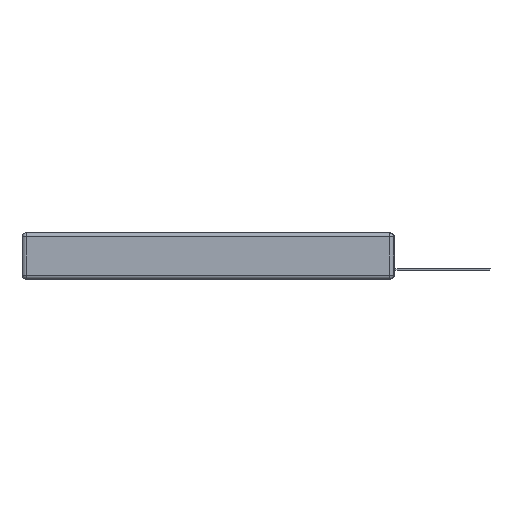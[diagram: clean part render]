
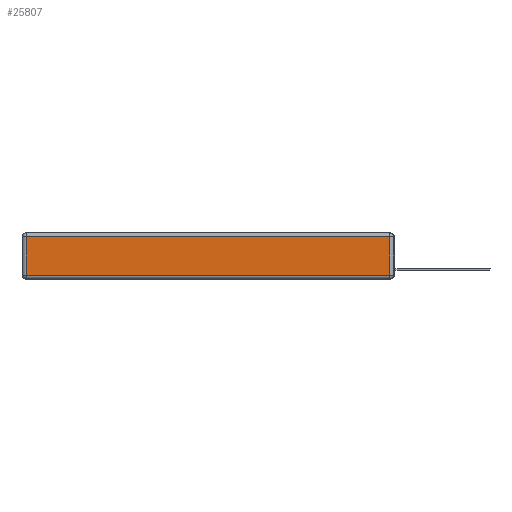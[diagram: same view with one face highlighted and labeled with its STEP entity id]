
A CAD part, left-side view. The second image highlights one B-rep face of the part: STEP entity #25807.
In plain terms, the highlighted planar face has unit normal (-1, 0, 0).
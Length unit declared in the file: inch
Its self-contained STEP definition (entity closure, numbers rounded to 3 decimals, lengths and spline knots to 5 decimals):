
#440 = DIRECTION ( 'NONE',  ( -1., 0., 0. ) ) ;
#2478 = PLANE ( 'NONE',  #12791 ) ;
#2831 = EDGE_CURVE ( 'NONE', #24040, #21944, #13257, .T. ) ;
#2901 = VERTEX_POINT ( 'NONE', #25821 ) ;
#3706 = VERTEX_POINT ( 'NONE', #24726 ) ;
#4555 = EDGE_CURVE ( 'NONE', #3706, #2901, #20381, .T. ) ;
#4625 = DIRECTION ( 'NONE',  ( 0., -1., 0. ) ) ;
#4902 = EDGE_CURVE ( 'NONE', #21944, #3706, #15594, .T. ) ;
#4913 = FACE_OUTER_BOUND ( 'NONE', #13018, .T. ) ;
#5460 = CARTESIAN_POINT ( 'NONE',  ( 0., 2.72, -0.343 ) ) ;
#5959 = VECTOR ( 'NONE', #4625, 39.37008 ) ;
#6176 = DIRECTION ( 'NONE',  ( 0., 1., 0. ) ) ;
#6598 = CARTESIAN_POINT ( 'NONE',  ( 0., 2.72, -0.313 ) ) ;
#7191 = ORIENTED_EDGE ( 'NONE', *, *, #4902, .T. ) ;
#12208 = VECTOR ( 'NONE', #6176, 39.37008 ) ;
#12253 = ORIENTED_EDGE ( 'NONE', *, *, #2831, .T. ) ;
#12481 = ORIENTED_EDGE ( 'NONE', *, *, #18104, .T. ) ;
#12791 = AXIS2_PLACEMENT_3D ( 'NONE', #19145, #440, #17092 ) ;
#12843 = CARTESIAN_POINT ( 'NONE',  ( 0., 0., -0.313 ) ) ;
#13018 = EDGE_LOOP ( 'NONE', ( #12253, #7191, #16410, #12481 ) ) ;
#13257 = LINE ( 'NONE', #12843, #5959 ) ;
#13679 = CARTESIAN_POINT ( 'NONE',  ( 0., 0.03, -0.343 ) ) ;
#14384 = CARTESIAN_POINT ( 'NONE',  ( 0., 2.75, -0.03 ) ) ;
#15530 = VECTOR ( 'NONE', #20470, 39.37008 ) ;
#15594 = LINE ( 'NONE', #13679, #18361 ) ;
#16410 = ORIENTED_EDGE ( 'NONE', *, *, #4555, .T. ) ;
#17092 = DIRECTION ( 'NONE',  ( 0., 0., 1. ) ) ;
#18065 = CARTESIAN_POINT ( 'NONE',  ( 0., 0.03, -0.313 ) ) ;
#18104 = EDGE_CURVE ( 'NONE', #2901, #24040, #21843, .T. ) ;
#18361 = VECTOR ( 'NONE', #26111, 39.37008 ) ;
#19145 = CARTESIAN_POINT ( 'NONE',  ( 0., 0., -0.343 ) ) ;
#20381 = LINE ( 'NONE', #14384, #12208 ) ;
#20470 = DIRECTION ( 'NONE',  ( 0., 0., -1. ) ) ;
#21843 = LINE ( 'NONE', #5460, #15530 ) ;
#21944 = VERTEX_POINT ( 'NONE', #18065 ) ;
#24040 = VERTEX_POINT ( 'NONE', #6598 ) ;
#24726 = CARTESIAN_POINT ( 'NONE',  ( 0., 0.03, -0.03 ) ) ;
#25807 = ADVANCED_FACE ( 'NONE', ( #4913 ), #2478, .T. ) ;
#25821 = CARTESIAN_POINT ( 'NONE',  ( 0., 2.72, -0.03 ) ) ;
#26111 = DIRECTION ( 'NONE',  ( 0., 0., 1. ) ) ;
